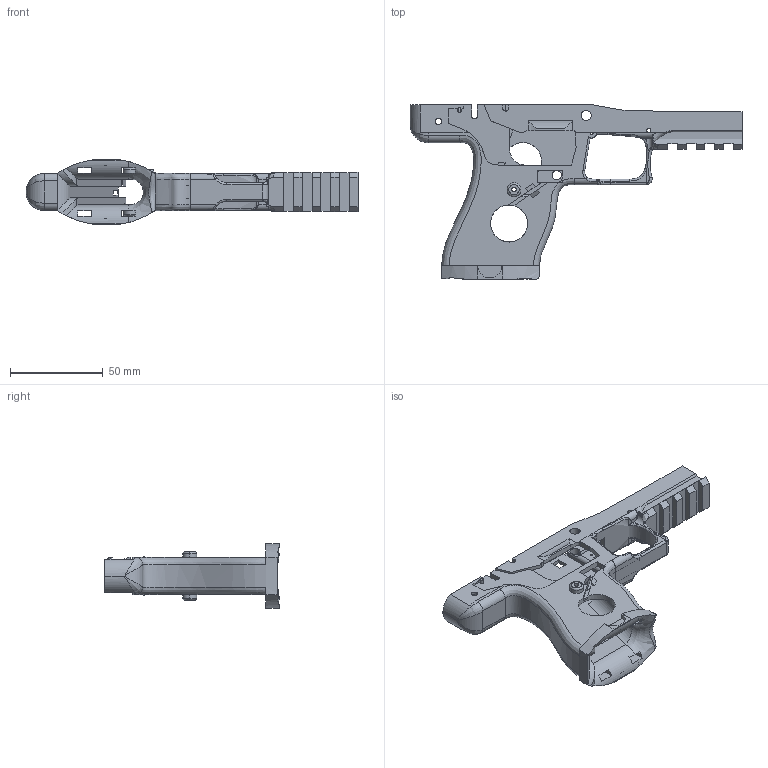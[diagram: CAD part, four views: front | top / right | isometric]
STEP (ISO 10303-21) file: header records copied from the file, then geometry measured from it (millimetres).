
FILE_DESCRIPTION (( 'STEP AP214' ), '1' );
FILE_NAME ('C9Frame.STEP', '2019-11-20T13:58:14', ( '' ), ( '' ), 'SwSTEP 2.0', 'SolidWorks 2017', '' );
FILE_SCHEMA (( 'AUTOMOTIVE_DESIGN' ));
Length unit declared in the file: millimetre
Products named in the file (1): C9Frame
Bounding box: 179 x 94 x 35 mm (x, y, z)
Volume: 73556.6 mm3; surface area: 38597.8 mm2
Topology: 1 solids, 1 shells, 414 faces, 1218 edges, 785 vertices
Faces by surface type: plane 222, cylinder 122, bspline 60, torus 10
Entity records: 18686 total; most frequent: CARTESIAN_POINT 8156, ORIENTED_EDGE 2424, DIRECTION 1895, EDGE_CURVE 1212, VERTEX_POINT 785, LINE 717, VECTOR 717, AXIS2_PLACEMENT_3D 589
